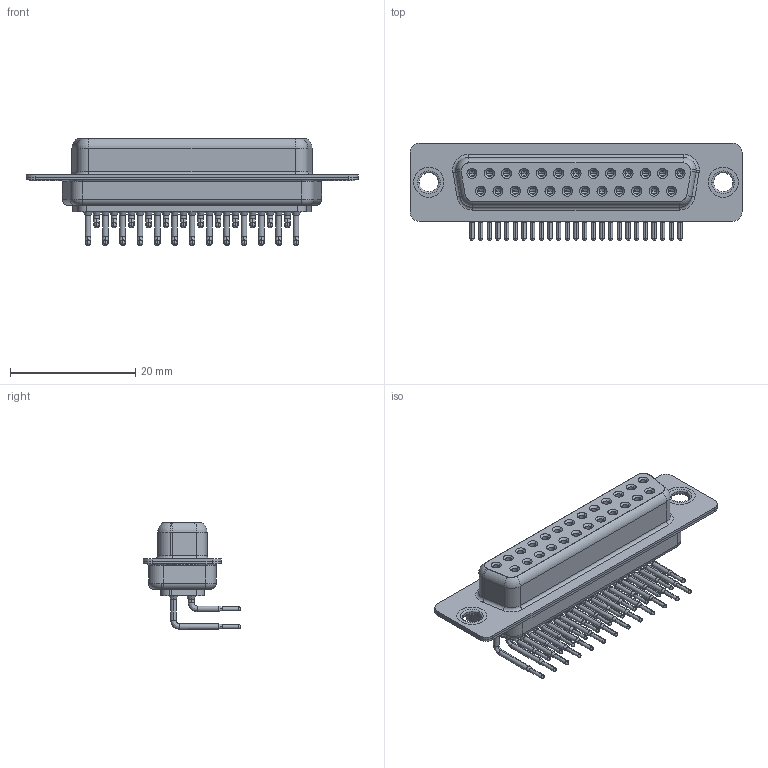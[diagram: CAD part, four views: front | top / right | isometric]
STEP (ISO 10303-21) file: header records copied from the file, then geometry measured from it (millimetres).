
FILE_DESCRIPTION (( 'STEP AP203' ), '1' );
FILE_NAME ('622-M25-360-GT1.STEP', '2018-09-24T21:56:29', ( '' ), ( '' ), 'SwSTEP 2.0', 'SolidWorks 2016', '' );
FILE_SCHEMA (( 'CONFIG_CONTROL_DESIGN' ));
Length unit declared in the file: millimetre
Products named in the file (7): 622M Housing_25 Contacts; 622M Shell Front_25 Contacts; 622M Shell Rear_25 Contacts; 622M Contact Row 1; 622M Contact Row 2; 622M Thru Hole Rivet; 622-M25-360-GT1
Assembly tree (30 placements, depth 2):
  622-M25-360-GT1
    622M Housing_25 Contacts
    622M Shell Front_25 Contacts
    622M Shell Rear_25 Contacts
    622M Contact Row 1  x13
    622M Contact Row 2  x12
    622M Thru Hole Rivet  x2
Bounding box: 53.05 x 15.6 x 17.09 mm (x, y, z)
Volume: 3773.1 mm3; surface area: 9351.8 mm2
Topology: 30 solids, 30 shells, 1578 faces, 3978 edges, 2496 vertices
Faces by surface type: cylinder 696, plane 442, cone 275, bspline 100, torus 65
Entity records: 20127 total; most frequent: DIRECTION 3573, CARTESIAN_POINT 3423, ORIENTED_EDGE 2938, AXIS2_PLACEMENT_3D 1502, EDGE_CURVE 1469, VERTEX_POINT 931, CIRCLE 839, EDGE_LOOP 790
